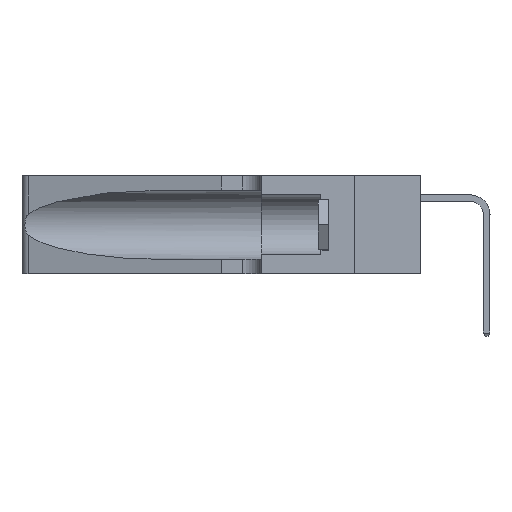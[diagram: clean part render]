
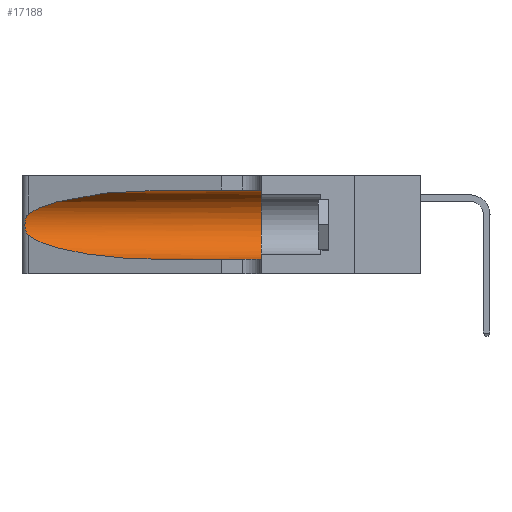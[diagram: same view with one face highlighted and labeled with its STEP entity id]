
A CAD part, left-side view. The second image highlights one B-rep face of the part: STEP entity #17188.
In plain terms, the highlighted cylindrical face has radius 3.308 mm (diameter 6.617 mm), a partial arc.
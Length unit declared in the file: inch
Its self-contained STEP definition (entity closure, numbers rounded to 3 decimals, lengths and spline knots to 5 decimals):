
#440 = CARTESIAN_POINT ( 'NONE',  ( 0.1305, 0.35, 0.31525 ) ) ;
#522 = CARTESIAN_POINT ( 'NONE',  ( 0.1305, 1.61858, 0.05475 ) ) ;
#943 = CARTESIAN_POINT ( 'NONE',  ( 0.26075, 1.23896, 0.19203 ) ) ;
#951 = CARTESIAN_POINT ( 'NONE',  ( 0.1305, 0.72297, 0.05475 ) ) ;
#1333 = CARTESIAN_POINT ( 'NONE',  ( 0.1305, 1.61858, 0.31525 ) ) ;
#1424 = CARTESIAN_POINT ( 'NONE',  ( 0.2373, 1.15595, 0.28018 ) ) ;
#1440 = B_SPLINE_CURVE_WITH_KNOTS ( 'NONE', 3,
 ( #9532, #15181, #16558, #8245, #17938, #9669, #943, #11070, #2447, #12471, #3911, #13842, #5377, #15245 ),
 .UNSPECIFIED., .F., .F.,
 ( 4, 2, 2, 2, 2, 2, 4 ),
 ( 0., 0.00027, 0.00053, 0.00107, 0.0016, 0.00187, 0.00214 ),
 .UNSPECIFIED. ) ;
#1591 = VECTOR ( 'NONE', #4906, 39.37008 ) ;
#1701 = CARTESIAN_POINT ( 'NONE',  ( 0.25487, 1.22718, 0.14631 ) ) ;
#1945 = CARTESIAN_POINT ( 'NONE',  ( 0.1305, 0.72297, 0.31525 ) ) ;
#2102 = ORIENTED_EDGE ( 'NONE', *, *, #14103, .T. ) ;
#2264 = ORIENTED_EDGE ( 'NONE', *, *, #17326, .F. ) ;
#2397 = LINE ( 'NONE', #1333, #13351 ) ;
#2447 = CARTESIAN_POINT ( 'NONE',  ( 0.26017, 1.23833, 0.17102 ) ) ;
#2725 = ORIENTED_EDGE ( 'NONE', *, *, #13620, .T. ) ;
#3886 = VERTEX_POINT ( 'NONE', #1701 ) ;
#3911 = CARTESIAN_POINT ( 'NONE',  ( 0.25789, 1.23486, 0.15765 ) ) ;
#3931 = CYLINDRICAL_SURFACE ( 'NONE', #11372, 0.13025 ) ;
#4217 = ORIENTED_EDGE ( 'NONE', *, *, #15673, .T. ) ;
#4605 = FACE_OUTER_BOUND ( 'NONE', #4766, .T. ) ;
#4612 = AXIS2_PLACEMENT_3D ( 'NONE', #6843, #16606, #8307 ) ;
#4766 = EDGE_LOOP ( 'NONE', ( #9717, #2725, #4217, #2102, #6173, #2264 ) ) ;
#4906 = DIRECTION ( 'NONE',  ( 0., -1., 0. ) ) ;
#5377 = CARTESIAN_POINT ( 'NONE',  ( 0.25555, 1.22993, 0.14849 ) ) ;
#5513 = VERTEX_POINT ( 'NONE', #8383 ) ;
#6173 = ORIENTED_EDGE ( 'NONE', *, *, #11450, .F. ) ;
#6843 = CARTESIAN_POINT ( 'NONE',  ( 0.1305, 0.35, 0.185 ) ) ;
#6856 =( BOUNDED_CURVE ( )  B_SPLINE_CURVE ( 3, ( #16565, #17943, #9676, #951 ),
 .UNSPECIFIED., .F., .T. ) 
 B_SPLINE_CURVE_WITH_KNOTS ( ( 4, 4 ),
 ( 3.44316, 4.71239 ),
 .UNSPECIFIED. ) 
 CURVE ( )  GEOMETRIC_REPRESENTATION_ITEM ( )  RATIONAL_B_SPLINE_CURVE ( ( 1., 0.87, 0.87, 1. ) ) 
 REPRESENTATION_ITEM ( '' )  );
#8210 = DIRECTION ( 'NONE',  ( 0., 0., -1. ) ) ;
#8245 = CARTESIAN_POINT ( 'NONE',  ( 0.25787, 1.23484, 0.2124 ) ) ;
#8307 = DIRECTION ( 'NONE',  ( 0., 0., 1. ) ) ;
#8383 = CARTESIAN_POINT ( 'NONE',  ( 0.1305, 0.72297, 0.05475 ) ) ;
#8418 = VERTEX_POINT ( 'NONE', #440 ) ;
#8421 = VERTEX_POINT ( 'NONE', #1945 ) ;
#8598 = CARTESIAN_POINT ( 'NONE',  ( 0.25487, 1.22718, 0.22369 ) ) ;
#8707 = CARTESIAN_POINT ( 'NONE',  ( 0.1305, 0.72297, 0.31525 ) ) ;
#9532 = CARTESIAN_POINT ( 'NONE',  ( 0.25487, 1.22718, 0.22369 ) ) ;
#9625 = CARTESIAN_POINT ( 'NONE',  ( 0.1305, 1.61858, 0.185 ) ) ;
#9669 = CARTESIAN_POINT ( 'NONE',  ( 0.26018, 1.23835, 0.19895 ) ) ;
#9676 = CARTESIAN_POINT ( 'NONE',  ( 0.18966, 0.96281, 0.05475 ) ) ;
#9717 = ORIENTED_EDGE ( 'NONE', *, *, #10355, .T. ) ;
#10130 = CARTESIAN_POINT ( 'NONE',  ( 0.18966, 0.96281, 0.31525 ) ) ;
#10313 = VERTEX_POINT ( 'NONE', #8598 ) ;
#10355 = EDGE_CURVE ( 'NONE', #8421, #10313, #17916, .T. ) ;
#11039 = DIRECTION ( 'NONE',  ( 0., -1., 0. ) ) ;
#11070 = CARTESIAN_POINT ( 'NONE',  ( 0.26075, 1.23896, 0.178 ) ) ;
#11372 = AXIS2_PLACEMENT_3D ( 'NONE', #9625, #11039, #8210 ) ;
#11450 = EDGE_CURVE ( 'NONE', #8418, #13266, #14019, .T. ) ;
#11464 = DIRECTION ( 'NONE',  ( 0., -1., 0. ) ) ;
#11522 = CARTESIAN_POINT ( 'NONE',  ( 0.25487, 1.22718, 0.22369 ) ) ;
#12471 = CARTESIAN_POINT ( 'NONE',  ( 0.25856, 1.23593, 0.16098 ) ) ;
#13266 = VERTEX_POINT ( 'NONE', #17104 ) ;
#13351 = VECTOR ( 'NONE', #11464, 39.37008 ) ;
#13620 = EDGE_CURVE ( 'NONE', #10313, #3886, #1440, .T. ) ;
#13842 = CARTESIAN_POINT ( 'NONE',  ( 0.25639, 1.23186, 0.15144 ) ) ;
#14019 = CIRCLE ( 'NONE', #4612, 0.13025 ) ;
#14103 = EDGE_CURVE ( 'NONE', #5513, #13266, #17132, .T. ) ;
#15181 = CARTESIAN_POINT ( 'NONE',  ( 0.25555, 1.22994, 0.2215 ) ) ;
#15245 = CARTESIAN_POINT ( 'NONE',  ( 0.25487, 1.22718, 0.14631 ) ) ;
#15673 = EDGE_CURVE ( 'NONE', #3886, #5513, #6856, .T. ) ;
#16558 = CARTESIAN_POINT ( 'NONE',  ( 0.25639, 1.23184, 0.21858 ) ) ;
#16565 = CARTESIAN_POINT ( 'NONE',  ( 0.25487, 1.22718, 0.14631 ) ) ;
#16606 = DIRECTION ( 'NONE',  ( 0., 1., 0. ) ) ;
#17104 = CARTESIAN_POINT ( 'NONE',  ( 0.1305, 0.35, 0.05475 ) ) ;
#17132 = LINE ( 'NONE', #522, #1591 ) ;
#17188 = ADVANCED_FACE ( 'NONE', ( #4605 ), #3931, .F. ) ;
#17326 = EDGE_CURVE ( 'NONE', #8421, #8418, #2397, .T. ) ;
#17916 =( BOUNDED_CURVE ( )  B_SPLINE_CURVE ( 3, ( #8707, #10130, #1424, #11522 ),
 .UNSPECIFIED., .F., .T. ) 
 B_SPLINE_CURVE_WITH_KNOTS ( ( 4, 4 ),
 ( 1.5708, 2.84003 ),
 .UNSPECIFIED. ) 
 CURVE ( )  GEOMETRIC_REPRESENTATION_ITEM ( )  RATIONAL_B_SPLINE_CURVE ( ( 1., 0.87, 0.87, 1. ) ) 
 REPRESENTATION_ITEM ( '' )  );
#17938 = CARTESIAN_POINT ( 'NONE',  ( 0.25854, 1.2359, 0.20912 ) ) ;
#17943 = CARTESIAN_POINT ( 'NONE',  ( 0.2373, 1.15595, 0.08982 ) ) ;
